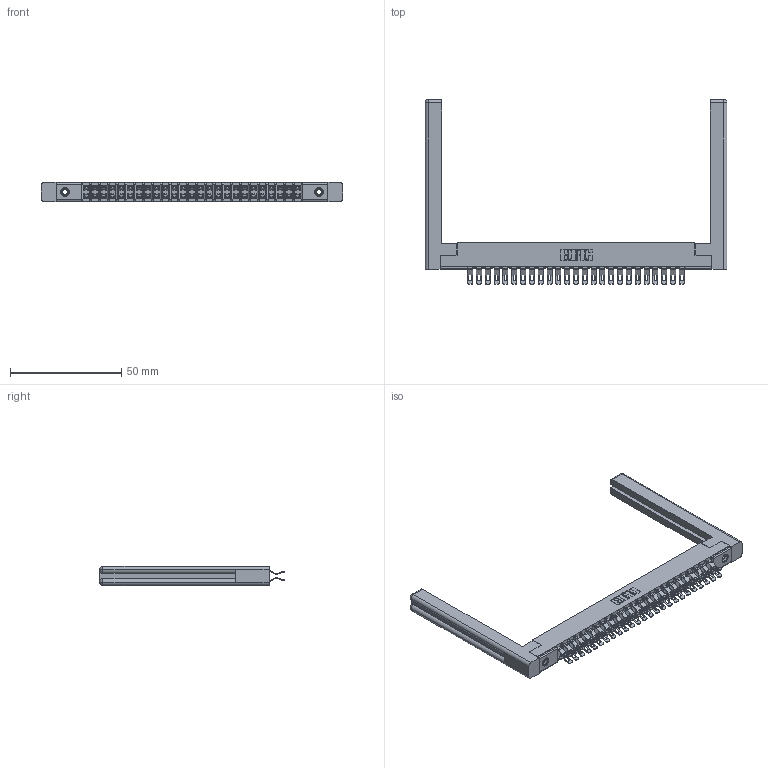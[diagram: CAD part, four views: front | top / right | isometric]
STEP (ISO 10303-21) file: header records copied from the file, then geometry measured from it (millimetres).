
FILE_DESCRIPTION (( 'STEP AP203' ), '1' );
FILE_NAME ('357-050-555-258.STEP', '2019-09-19T02:52:45', ( '' ), ( '' ), 'SwSTEP 2.0', 'SolidWorks 2016', '' );
FILE_SCHEMA (( 'CONFIG_CONTROL_DESIGN' ));
Length unit declared in the file: inch
Products named in the file (5): 307-290-001_555; 307 Part_.156 Dia Mounting Holes; 307-220-058; 345-250-001_345-250-001-102; 357-050-555-258
Assembly tree (55 placements, depth 2):
  357-050-555-258
    307 Part_.156 Dia Mounting Holes
    307-290-001_555  x50
    307-220-058  x2
    345-250-001_345-250-001-102  x2
Bounding box: 135.69 x 83.06 x 8.71 mm (x, y, z)
Volume: 16710.6 mm3; surface area: 22007.3 mm2
Topology: 55 solids, 55 shells, 3336 faces, 9727 edges, 6334 vertices
Faces by surface type: plane 1854, cylinder 1406, sphere 52, torus 12, cone 12
Entity records: 27498 total; most frequent: CARTESIAN_POINT 4528, ORIENTED_EDGE 4430, DIRECTION 4407, EDGE_CURVE 2215, LINE 1677, VECTOR 1677, VERTEX_POINT 1432, AXIS2_PLACEMENT_3D 1365
